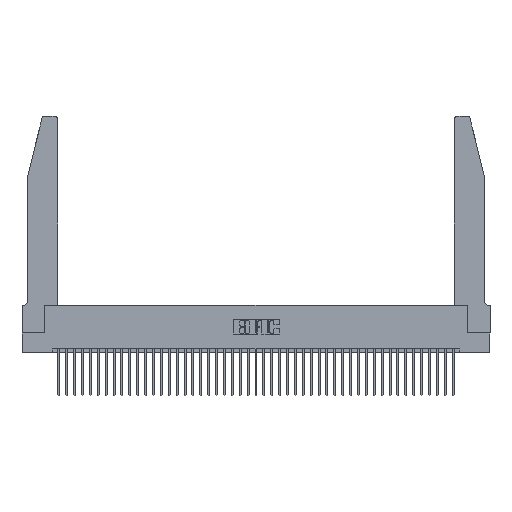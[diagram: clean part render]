
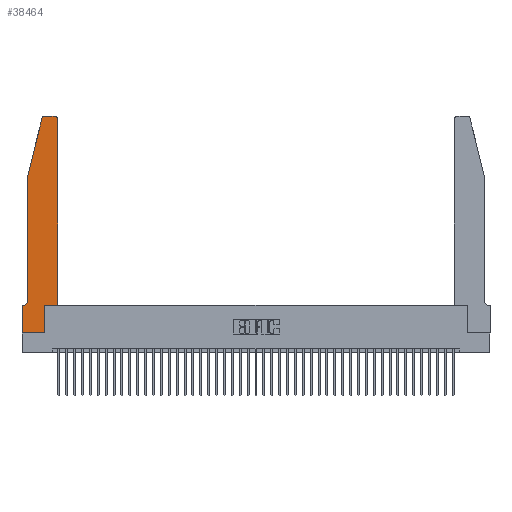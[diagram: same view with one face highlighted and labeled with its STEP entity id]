
A CAD part, top view. The second image highlights one B-rep face of the part: STEP entity #38464.
In plain terms, the highlighted planar face has unit normal (0, 0, 1).
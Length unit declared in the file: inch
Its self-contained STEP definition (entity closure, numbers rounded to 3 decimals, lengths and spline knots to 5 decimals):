
#522 = CARTESIAN_POINT ( 'NONE',  ( 0.4505, 0.35, 0.37 ) ) ;
#902 = LINE ( 'NONE', #21107, #17900 ) ;
#1746 = DIRECTION ( 'NONE',  ( 0., 1., 0. ) ) ;
#1985 = ORIENTED_EDGE ( 'NONE', *, *, #23923, .T. ) ;
#2230 = DIRECTION ( 'NONE',  ( -1., 0., 0. ) ) ;
#2616 = VECTOR ( 'NONE', #41020, 39.37008 ) ;
#2742 = ORIENTED_EDGE ( 'NONE', *, *, #38719, .T. ) ;
#2870 = EDGE_CURVE ( 'NONE', #23882, #8413, #13792, .T. ) ;
#3296 = ORIENTED_EDGE ( 'NONE', *, *, #2870, .T. ) ;
#3552 = LINE ( 'NONE', #8482, #38283 ) ;
#4123 = FACE_OUTER_BOUND ( 'NONE', #33812, .T. ) ;
#4267 = DIRECTION ( 'NONE',  ( 0., 0., 1. ) ) ;
#4380 = ORIENTED_EDGE ( 'NONE', *, *, #37296, .T. ) ;
#5761 = DIRECTION ( 'NONE',  ( 0., 0., 1. ) ) ;
#6585 = EDGE_CURVE ( 'NONE', #31255, #15619, #18790, .T. ) ;
#6766 = CARTESIAN_POINT ( 'NONE',  ( 0.4205, 2.75, 0.37 ) ) ;
#7389 = CARTESIAN_POINT ( 'NONE',  ( 0., 0., 0.37 ) ) ;
#8413 = VERTEX_POINT ( 'NONE', #37800 ) ;
#8482 = CARTESIAN_POINT ( 'NONE',  ( 0., 0., 0.37 ) ) ;
#8512 = ORIENTED_EDGE ( 'NONE', *, *, #37289, .T. ) ;
#8968 = CARTESIAN_POINT ( 'NONE',  ( 0.0755, 2., 0.37 ) ) ;
#9149 = ORIENTED_EDGE ( 'NONE', *, *, #23875, .T. ) ;
#9937 = EDGE_CURVE ( 'NONE', #21862, #38068, #902, .T. ) ;
#10505 = EDGE_CURVE ( 'NONE', #21447, #41630, #14688, .T. ) ;
#11704 = CARTESIAN_POINT ( 'NONE',  ( 0., 0., 0.37 ) ) ;
#12097 = AXIS2_PLACEMENT_3D ( 'NONE', #25899, #5761, #29266 ) ;
#12163 = ORIENTED_EDGE ( 'NONE', *, *, #10505, .T. ) ;
#12373 = CARTESIAN_POINT ( 'NONE',  ( 0.0755, 2., 0.37 ) ) ;
#12383 = VECTOR ( 'NONE', #42248, 39.37008 ) ;
#13119 = LINE ( 'NONE', #28732, #22075 ) ;
#13431 = LINE ( 'NONE', #28776, #12383 ) ;
#13792 = LINE ( 'NONE', #522, #2616 ) ;
#13919 = ORIENTED_EDGE ( 'NONE', *, *, #31726, .T. ) ;
#14688 = LINE ( 'NONE', #40930, #24644 ) ;
#14873 = CARTESIAN_POINT ( 'NONE',  ( 0.284, 2.75, 0.37 ) ) ;
#15088 = CARTESIAN_POINT ( 'NONE',  ( 0.0755, 0.35, 0.37 ) ) ;
#15612 = ORIENTED_EDGE ( 'NONE', *, *, #17107, .T. ) ;
#15619 = VERTEX_POINT ( 'NONE', #31283 ) ;
#15622 = CARTESIAN_POINT ( 'NONE',  ( 0.4505, 0.35, 0.37 ) ) ;
#15755 = VERTEX_POINT ( 'NONE', #25279 ) ;
#15864 = ORIENTED_EDGE ( 'NONE', *, *, #9937, .T. ) ;
#17107 = EDGE_CURVE ( 'NONE', #41630, #24191, #27883, .T. ) ;
#17372 = CARTESIAN_POINT ( 'NONE',  ( 0., 0.35, 0.37 ) ) ;
#17541 = DIRECTION ( 'NONE',  ( -1., 0., 0. ) ) ;
#17900 = VECTOR ( 'NONE', #28089, 39.37008 ) ;
#18667 = DIRECTION ( 'NONE',  ( 1., 0., 0. ) ) ;
#18790 = LINE ( 'NONE', #15088, #35526 ) ;
#19062 = VERTEX_POINT ( 'NONE', #30598 ) ;
#19063 = AXIS2_PLACEMENT_3D ( 'NONE', #24460, #4267, #27820 ) ;
#20621 = CIRCLE ( 'NONE', #36160, 0.07 ) ;
#20738 = DIRECTION ( 'NONE',  ( 1., 0., 0. ) ) ;
#21107 = CARTESIAN_POINT ( 'NONE',  ( 0.0755, 2., 0.37 ) ) ;
#21330 = LINE ( 'NONE', #12373, #37019 ) ;
#21447 = VERTEX_POINT ( 'NONE', #6766 ) ;
#21847 = DIRECTION ( 'NONE',  ( -1., 0., 0. ) ) ;
#21862 = VERTEX_POINT ( 'NONE', #8968 ) ;
#22075 = VECTOR ( 'NONE', #1746, 39.37008 ) ;
#22514 = DIRECTION ( 'NONE',  ( 0., 0., -1. ) ) ;
#23754 = CIRCLE ( 'NONE', #19063, 0.03 ) ;
#23875 = EDGE_CURVE ( 'NONE', #19062, #23882, #13431, .T. ) ;
#23882 = VERTEX_POINT ( 'NONE', #15622 ) ;
#23923 = EDGE_CURVE ( 'NONE', #24191, #21862, #21330, .T. ) ;
#24191 = VERTEX_POINT ( 'NONE', #42092 ) ;
#24460 = CARTESIAN_POINT ( 'NONE',  ( 0.4205, 2.72, 0.37 ) ) ;
#24644 = VECTOR ( 'NONE', #17541, 39.37008 ) ;
#25279 = CARTESIAN_POINT ( 'NONE',  ( 0.2865, 0., 0.37 ) ) ;
#25899 = CARTESIAN_POINT ( 'NONE',  ( 0.284, 2.72, 0.37 ) ) ;
#26030 = EDGE_CURVE ( 'NONE', #38068, #31255, #20621, .T. ) ;
#26127 = CARTESIAN_POINT ( 'NONE',  ( 0.0055, 0.35, 0.37 ) ) ;
#27278 = PLANE ( 'NONE',  #29974 ) ;
#27820 = DIRECTION ( 'NONE',  ( 1., 0., 0. ) ) ;
#27883 = CIRCLE ( 'NONE', #12097, 0.03 ) ;
#28089 = DIRECTION ( 'NONE',  ( 0., -1., 0. ) ) ;
#28398 = ORIENTED_EDGE ( 'NONE', *, *, #26030, .T. ) ;
#28732 = CARTESIAN_POINT ( 'NONE',  ( 0.2865, 0.35, 0.37 ) ) ;
#28776 = CARTESIAN_POINT ( 'NONE',  ( 0.4505, 0.35, 0.37 ) ) ;
#29266 = DIRECTION ( 'NONE',  ( 1., 0., 0. ) ) ;
#29974 = AXIS2_PLACEMENT_3D ( 'NONE', #17372, #40750, #20738 ) ;
#30598 = CARTESIAN_POINT ( 'NONE',  ( 0.2865, 0.35, 0.37 ) ) ;
#31255 = VERTEX_POINT ( 'NONE', #26127 ) ;
#31283 = CARTESIAN_POINT ( 'NONE',  ( 0., 0.35, 0.37 ) ) ;
#31586 = VECTOR ( 'NONE', #37783, 39.37008 ) ;
#31726 = EDGE_CURVE ( 'NONE', #15755, #19062, #13119, .T. ) ;
#33812 = EDGE_LOOP ( 'NONE', ( #12163, #15612, #1985, #15864, #28398, #38502, #8512, #2742, #13919, #9149, #3296, #4380 ) ) ;
#35526 = VECTOR ( 'NONE', #21847, 39.37008 ) ;
#35816 = DIRECTION ( 'NONE',  ( -0.239, -0.971, 0. ) ) ;
#36160 = AXIS2_PLACEMENT_3D ( 'NONE', #42526, #22514, #2230 ) ;
#37019 = VECTOR ( 'NONE', #35816, 39.37008 ) ;
#37289 = EDGE_CURVE ( 'NONE', #15619, #43557, #40498, .T. ) ;
#37296 = EDGE_CURVE ( 'NONE', #8413, #21447, #23754, .T. ) ;
#37783 = DIRECTION ( 'NONE',  ( 0., -1., 0. ) ) ;
#37800 = CARTESIAN_POINT ( 'NONE',  ( 0.4505, 2.72, 0.37 ) ) ;
#38068 = VERTEX_POINT ( 'NONE', #41971 ) ;
#38283 = VECTOR ( 'NONE', #18667, 39.37008 ) ;
#38464 = ADVANCED_FACE ( 'NONE', ( #4123 ), #27278, .T. ) ;
#38502 = ORIENTED_EDGE ( 'NONE', *, *, #6585, .T. ) ;
#38719 = EDGE_CURVE ( 'NONE', #43557, #15755, #3552, .T. ) ;
#40498 = LINE ( 'NONE', #7389, #31586 ) ;
#40750 = DIRECTION ( 'NONE',  ( 0., 0., 1. ) ) ;
#40930 = CARTESIAN_POINT ( 'NONE',  ( 0.2605, 2.75, 0.37 ) ) ;
#41020 = DIRECTION ( 'NONE',  ( 0., 1., 0. ) ) ;
#41630 = VERTEX_POINT ( 'NONE', #14873 ) ;
#41971 = CARTESIAN_POINT ( 'NONE',  ( 0.0755, 0.42, 0.37 ) ) ;
#42092 = CARTESIAN_POINT ( 'NONE',  ( 0.25487, 2.72718, 0.37 ) ) ;
#42248 = DIRECTION ( 'NONE',  ( 1., 0., 0. ) ) ;
#42526 = CARTESIAN_POINT ( 'NONE',  ( 0.0055, 0.42, 0.37 ) ) ;
#43557 = VERTEX_POINT ( 'NONE', #11704 ) ;
